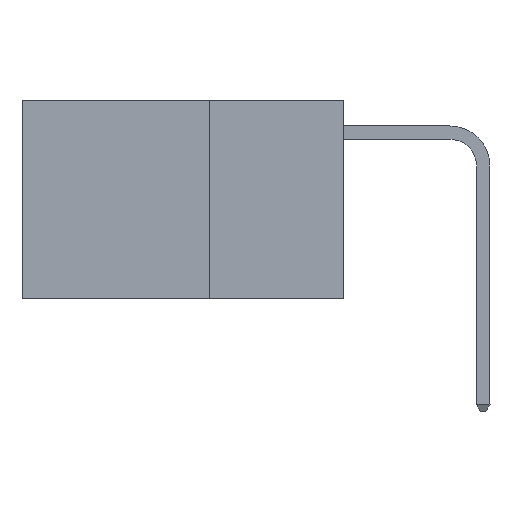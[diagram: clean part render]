
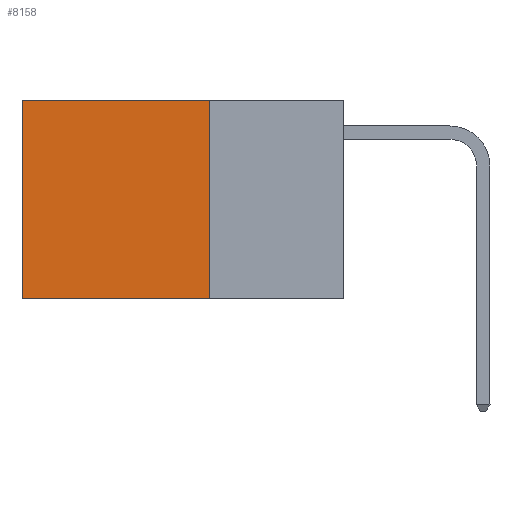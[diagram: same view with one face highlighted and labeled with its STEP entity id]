
A CAD part, left-side view. The second image highlights one B-rep face of the part: STEP entity #8158.
In plain terms, the highlighted planar face has unit normal (-1, 0, 0).
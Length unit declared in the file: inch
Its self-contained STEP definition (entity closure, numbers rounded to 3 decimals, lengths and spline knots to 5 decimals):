
#106 = LINE ( 'NONE', #7062, #9538 ) ;
#998 = EDGE_CURVE ( 'NONE', #1990, #10824, #106, .T. ) ;
#1362 = CARTESIAN_POINT ( 'NONE',  ( 0.2625, 0.6, -0.37 ) ) ;
#1699 = ORIENTED_EDGE ( 'NONE', *, *, #15060, .T. ) ;
#1990 = VERTEX_POINT ( 'NONE', #7722 ) ;
#2748 = EDGE_CURVE ( 'NONE', #10824, #14016, #9322, .T. ) ;
#2765 = VECTOR ( 'NONE', #10688, 39.37008 ) ;
#4808 = CARTESIAN_POINT ( 'NONE',  ( 0.2625, 0.25, -0.37 ) ) ;
#4850 = EDGE_LOOP ( 'NONE', ( #1699, #14408, #5767, #9044 ) ) ;
#5230 = VECTOR ( 'NONE', #14921, 39.37008 ) ;
#5767 = ORIENTED_EDGE ( 'NONE', *, *, #998, .F. ) ;
#6156 = VERTEX_POINT ( 'NONE', #15115 ) ;
#7062 = CARTESIAN_POINT ( 'NONE',  ( 0.2625, 0.25, 0. ) ) ;
#7139 = DIRECTION ( 'NONE',  ( 1., 0., 0. ) ) ;
#7569 = CARTESIAN_POINT ( 'NONE',  ( 0.2625, 0.25, -0.37 ) ) ;
#7722 = CARTESIAN_POINT ( 'NONE',  ( 0.2625, 0.25, 0. ) ) ;
#8038 = CARTESIAN_POINT ( 'NONE',  ( 0.2625, 0.25, 0. ) ) ;
#8158 = ADVANCED_FACE ( 'NONE', ( #8231 ), #11808, .F. ) ;
#8231 = FACE_OUTER_BOUND ( 'NONE', #4850, .T. ) ;
#9044 = ORIENTED_EDGE ( 'NONE', *, *, #14899, .T. ) ;
#9096 = AXIS2_PLACEMENT_3D ( 'NONE', #14124, #7139, #15245 ) ;
#9268 = DIRECTION ( 'NONE',  ( 0., 0., -1. ) ) ;
#9270 = LINE ( 'NONE', #8038, #5230 ) ;
#9322 = LINE ( 'NONE', #4808, #2765 ) ;
#9512 = CARTESIAN_POINT ( 'NONE',  ( 0.2625, 0.6, 0. ) ) ;
#9538 = VECTOR ( 'NONE', #9268, 39.37008 ) ;
#10688 = DIRECTION ( 'NONE',  ( 0., 1., 0. ) ) ;
#10824 = VERTEX_POINT ( 'NONE', #7569 ) ;
#11808 = PLANE ( 'NONE',  #9096 ) ;
#12461 = LINE ( 'NONE', #9512, #15147 ) ;
#12946 = DIRECTION ( 'NONE',  ( 0., 0., -1. ) ) ;
#14016 = VERTEX_POINT ( 'NONE', #1362 ) ;
#14124 = CARTESIAN_POINT ( 'NONE',  ( 0.2625, 0.25, 0. ) ) ;
#14408 = ORIENTED_EDGE ( 'NONE', *, *, #2748, .F. ) ;
#14899 = EDGE_CURVE ( 'NONE', #1990, #6156, #9270, .T. ) ;
#14921 = DIRECTION ( 'NONE',  ( 0., 1., 0. ) ) ;
#15060 = EDGE_CURVE ( 'NONE', #6156, #14016, #12461, .T. ) ;
#15115 = CARTESIAN_POINT ( 'NONE',  ( 0.2625, 0.6, 0. ) ) ;
#15147 = VECTOR ( 'NONE', #12946, 39.37008 ) ;
#15245 = DIRECTION ( 'NONE',  ( 0., 0., -1. ) ) ;
